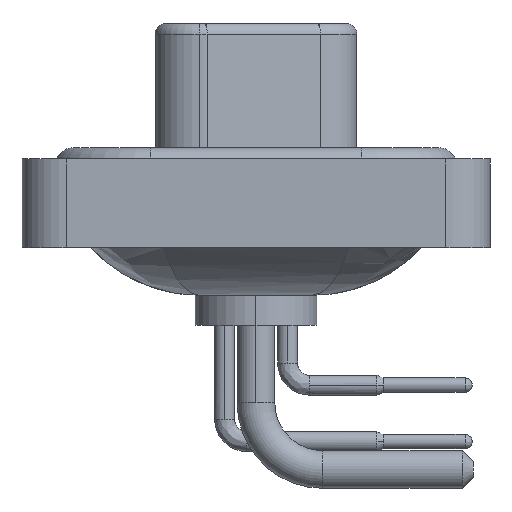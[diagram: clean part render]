
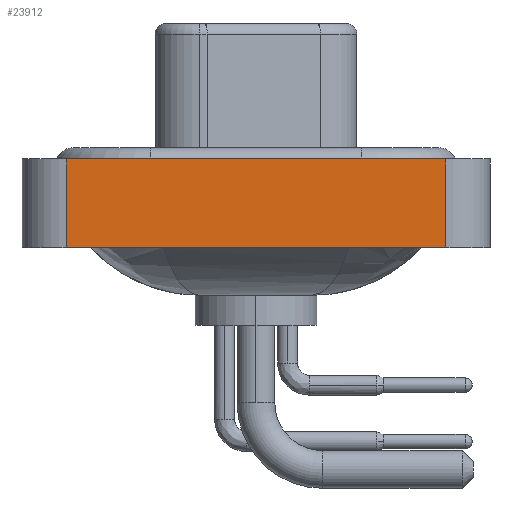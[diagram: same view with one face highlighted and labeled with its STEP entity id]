
A CAD part, left-side view. The second image highlights one B-rep face of the part: STEP entity #23912.
In plain terms, the highlighted planar face has unit normal (-1, 0, 0).
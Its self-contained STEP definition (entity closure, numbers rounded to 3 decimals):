
#410 = VERTEX_POINT ( 'NONE', #17714 ) ;
#736 = VECTOR ( 'NONE', #2845, 1000. ) ;
#2114 = DIRECTION ( 'NONE',  ( -1., 0., 0. ) ) ;
#2248 = CARTESIAN_POINT ( 'NONE',  ( -7.35, -8.55, -3.6 ) ) ;
#2705 = LINE ( 'NONE', #11008, #736 ) ;
#2845 = DIRECTION ( 'NONE',  ( 0., -1., 0. ) ) ;
#4409 = EDGE_CURVE ( 'NONE', #4713, #7449, #22270, .T. ) ;
#4626 = CARTESIAN_POINT ( 'NONE',  ( -7.35, -8.55, -3.6 ) ) ;
#4713 = VERTEX_POINT ( 'NONE', #13144 ) ;
#6522 = AXIS2_PLACEMENT_3D ( 'NONE', #2248, #2114, #12757 ) ;
#6724 = LINE ( 'NONE', #8938, #12203 ) ;
#7449 = VERTEX_POINT ( 'NONE', #4626 ) ;
#7505 = VECTOR ( 'NONE', #26104, 1000. ) ;
#8938 = CARTESIAN_POINT ( 'NONE',  ( -7.35, -8.55, -3.6 ) ) ;
#9545 = CARTESIAN_POINT ( 'NONE',  ( -7.35, 8.55, -3.6 ) ) ;
#9760 = CARTESIAN_POINT ( 'NONE',  ( -7.35, -8.55, -3.6 ) ) ;
#9977 = EDGE_LOOP ( 'NONE', ( #24682, #22541, #21613, #12890 ) ) ;
#10110 = EDGE_CURVE ( 'NONE', #4713, #410, #19985, .T. ) ;
#10313 = VECTOR ( 'NONE', #11455, 1000. ) ;
#11008 = CARTESIAN_POINT ( 'NONE',  ( -7.35, -8.55, 0.4 ) ) ;
#11455 = DIRECTION ( 'NONE',  ( 0., 0., 1. ) ) ;
#11926 = FACE_OUTER_BOUND ( 'NONE', #9977, .T. ) ;
#12203 = VECTOR ( 'NONE', #23793, 1000. ) ;
#12757 = DIRECTION ( 'NONE',  ( 0., 0., 1. ) ) ;
#12890 = ORIENTED_EDGE ( 'NONE', *, *, #4409, .T. ) ;
#13144 = CARTESIAN_POINT ( 'NONE',  ( -7.35, 8.55, -3.6 ) ) ;
#16820 = VERTEX_POINT ( 'NONE', #21148 ) ;
#17714 = CARTESIAN_POINT ( 'NONE',  ( -7.35, 8.55, 0.4 ) ) ;
#19985 = LINE ( 'NONE', #9545, #10313 ) ;
#21148 = CARTESIAN_POINT ( 'NONE',  ( -7.35, -8.55, 0.4 ) ) ;
#21613 = ORIENTED_EDGE ( 'NONE', *, *, #10110, .F. ) ;
#21930 = EDGE_CURVE ( 'NONE', #410, #16820, #2705, .T. ) ;
#21960 = EDGE_CURVE ( 'NONE', #7449, #16820, #6724, .T. ) ;
#22106 = PLANE ( 'NONE',  #6522 ) ;
#22270 = LINE ( 'NONE', #9760, #7505 ) ;
#22541 = ORIENTED_EDGE ( 'NONE', *, *, #21930, .F. ) ;
#23793 = DIRECTION ( 'NONE',  ( 0., 0., 1. ) ) ;
#23912 = ADVANCED_FACE ( 'NONE', ( #11926 ), #22106, .T. ) ;
#24682 = ORIENTED_EDGE ( 'NONE', *, *, #21960, .T. ) ;
#26104 = DIRECTION ( 'NONE',  ( 0., -1., 0. ) ) ;
